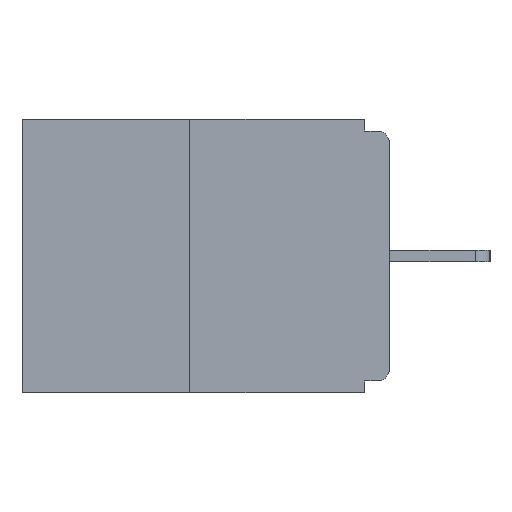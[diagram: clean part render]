
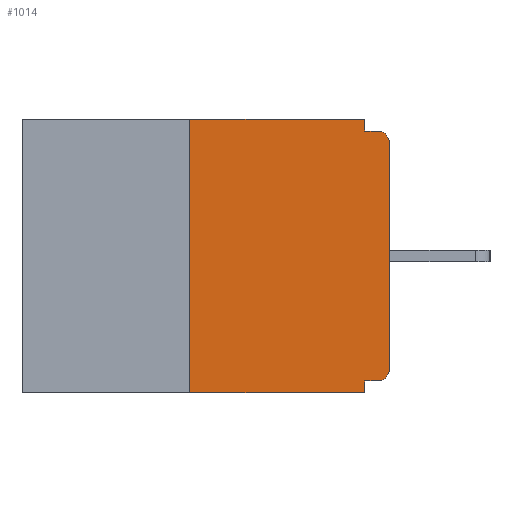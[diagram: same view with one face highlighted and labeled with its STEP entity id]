
A CAD part, left-side view. The second image highlights one B-rep face of the part: STEP entity #1014.
In plain terms, the highlighted planar face has unit normal (-1, 0, 0).
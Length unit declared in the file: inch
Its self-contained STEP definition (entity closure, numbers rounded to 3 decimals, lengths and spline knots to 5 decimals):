
#24 = AXIS2_PLACEMENT_3D ( 'NONE', #11627, #16337, #543 ) ;
#31 = PLANE ( 'NONE',  #9150 ) ;
#236 = VERTEX_POINT ( 'NONE', #1816 ) ;
#464 = DIRECTION ( 'NONE',  ( 0., 1., 0. ) ) ;
#543 = DIRECTION ( 'NONE',  ( 0., 0., -1. ) ) ;
#619 = VECTOR ( 'NONE', #464, 39.37008 ) ;
#634 = ORIENTED_EDGE ( 'NONE', *, *, #17461, .F. ) ;
#799 = VECTOR ( 'NONE', #11087, 39.37008 ) ;
#919 = CARTESIAN_POINT ( 'NONE',  ( 0., 0., -0.015 ) ) ;
#1014 = ADVANCED_FACE ( 'NONE', ( #18389 ), #31, .F. ) ;
#1371 = VERTEX_POINT ( 'NONE', #19399 ) ;
#1380 = CARTESIAN_POINT ( 'NONE',  ( 0., 0.46, -0.343 ) ) ;
#1462 = CARTESIAN_POINT ( 'NONE',  ( 0., 0.031, -0.343 ) ) ;
#1732 = VECTOR ( 'NONE', #15837, 39.37008 ) ;
#1816 = CARTESIAN_POINT ( 'NONE',  ( 0., 0.015, -0.328 ) ) ;
#1890 = DIRECTION ( 'NONE',  ( 0., 0., 1. ) ) ;
#2006 = CARTESIAN_POINT ( 'NONE',  ( 0., 0., -0.328 ) ) ;
#2594 = LINE ( 'NONE', #919, #13530 ) ;
#2870 = EDGE_CURVE ( 'NONE', #16396, #18746, #8162, .T. ) ;
#2949 = CARTESIAN_POINT ( 'NONE',  ( 0., 0.46, 0. ) ) ;
#3344 = CARTESIAN_POINT ( 'NONE',  ( 0., 0.25, -0.343 ) ) ;
#4379 = DIRECTION ( 'NONE',  ( 0., -1., 0. ) ) ;
#4965 = CARTESIAN_POINT ( 'NONE',  ( 0., 0., 0. ) ) ;
#5162 = EDGE_LOOP ( 'NONE', ( #634, #14019, #11768, #8451, #11698, #6774, #19658, #11489, #8100, #15790 ) ) ;
#5183 = CARTESIAN_POINT ( 'NONE',  ( 0., 0.031, -0.015 ) ) ;
#5186 = CIRCLE ( 'NONE', #12373, 0.015 ) ;
#6774 = ORIENTED_EDGE ( 'NONE', *, *, #8392, .T. ) ;
#6930 = DIRECTION ( 'NONE',  ( 0., 0., -1. ) ) ;
#7028 = CARTESIAN_POINT ( 'NONE',  ( 0., 0.031, 0. ) ) ;
#7117 = CARTESIAN_POINT ( 'NONE',  ( 0., 0.015, -0.015 ) ) ;
#7536 = VERTEX_POINT ( 'NONE', #10332 ) ;
#7780 = CARTESIAN_POINT ( 'NONE',  ( 0., 0.46, 0. ) ) ;
#8011 = LINE ( 'NONE', #1380, #1732 ) ;
#8100 = ORIENTED_EDGE ( 'NONE', *, *, #20112, .F. ) ;
#8162 = LINE ( 'NONE', #12700, #799 ) ;
#8213 = EDGE_CURVE ( 'NONE', #1371, #7536, #9480, .T. ) ;
#8258 = VECTOR ( 'NONE', #6930, 39.37008 ) ;
#8392 = EDGE_CURVE ( 'NONE', #236, #1371, #5186, .T. ) ;
#8451 = ORIENTED_EDGE ( 'NONE', *, *, #12208, .F. ) ;
#8612 = DIRECTION ( 'NONE',  ( 0., 0., -1. ) ) ;
#8815 = CARTESIAN_POINT ( 'NONE',  ( 0., 0.031, -0.328 ) ) ;
#9036 = DIRECTION ( 'NONE',  ( 1., 0., 0. ) ) ;
#9150 = AXIS2_PLACEMENT_3D ( 'NONE', #7780, #9036, #20032 ) ;
#9480 = LINE ( 'NONE', #4965, #18611 ) ;
#9833 = VERTEX_POINT ( 'NONE', #1462 ) ;
#10052 = DIRECTION ( 'NONE',  ( 0., -1., 0. ) ) ;
#10144 = CARTESIAN_POINT ( 'NONE',  ( 0., 0.031, 0. ) ) ;
#10171 = LINE ( 'NONE', #16431, #11483 ) ;
#10332 = CARTESIAN_POINT ( 'NONE',  ( 0., 0., -0.03 ) ) ;
#10763 = VERTEX_POINT ( 'NONE', #5183 ) ;
#10832 = EDGE_CURVE ( 'NONE', #236, #18244, #15948, .T. ) ;
#11087 = DIRECTION ( 'NONE',  ( 0., 0., 1. ) ) ;
#11332 = VERTEX_POINT ( 'NONE', #10144 ) ;
#11483 = VECTOR ( 'NONE', #8612, 39.37008 ) ;
#11489 = ORIENTED_EDGE ( 'NONE', *, *, #12169, .T. ) ;
#11627 = CARTESIAN_POINT ( 'NONE',  ( 0., 0.015, -0.03 ) ) ;
#11698 = ORIENTED_EDGE ( 'NONE', *, *, #10832, .F. ) ;
#11768 = ORIENTED_EDGE ( 'NONE', *, *, #16404, .T. ) ;
#12169 = EDGE_CURVE ( 'NONE', #7536, #13231, #17032, .T. ) ;
#12208 = EDGE_CURVE ( 'NONE', #18244, #9833, #10171, .T. ) ;
#12211 = CARTESIAN_POINT ( 'NONE',  ( 0., 0.015, -0.313 ) ) ;
#12373 = AXIS2_PLACEMENT_3D ( 'NONE', #12211, #13805, #16621 ) ;
#12562 = CARTESIAN_POINT ( 'NONE',  ( 0., 0.25, 0. ) ) ;
#12700 = CARTESIAN_POINT ( 'NONE',  ( 0., 0.25, 0. ) ) ;
#13231 = VERTEX_POINT ( 'NONE', #7117 ) ;
#13530 = VECTOR ( 'NONE', #10052, 39.37008 ) ;
#13805 = DIRECTION ( 'NONE',  ( -1., 0., 0. ) ) ;
#14019 = ORIENTED_EDGE ( 'NONE', *, *, #2870, .F. ) ;
#15790 = ORIENTED_EDGE ( 'NONE', *, *, #19254, .F. ) ;
#15837 = DIRECTION ( 'NONE',  ( 0., -1., 0. ) ) ;
#15948 = LINE ( 'NONE', #2006, #619 ) ;
#16192 = LINE ( 'NONE', #7028, #8258 ) ;
#16337 = DIRECTION ( 'NONE',  ( -1., 0., 0. ) ) ;
#16396 = VERTEX_POINT ( 'NONE', #3344 ) ;
#16404 = EDGE_CURVE ( 'NONE', #16396, #9833, #8011, .T. ) ;
#16431 = CARTESIAN_POINT ( 'NONE',  ( 0., 0.031, -0.343 ) ) ;
#16621 = DIRECTION ( 'NONE',  ( 0., 0., -1. ) ) ;
#17032 = CIRCLE ( 'NONE', #24, 0.015 ) ;
#17461 = EDGE_CURVE ( 'NONE', #18746, #11332, #18420, .T. ) ;
#17502 = VECTOR ( 'NONE', #4379, 39.37008 ) ;
#18244 = VERTEX_POINT ( 'NONE', #8815 ) ;
#18389 = FACE_OUTER_BOUND ( 'NONE', #5162, .T. ) ;
#18420 = LINE ( 'NONE', #2949, #17502 ) ;
#18611 = VECTOR ( 'NONE', #1890, 39.37008 ) ;
#18746 = VERTEX_POINT ( 'NONE', #12562 ) ;
#19254 = EDGE_CURVE ( 'NONE', #11332, #10763, #16192, .T. ) ;
#19399 = CARTESIAN_POINT ( 'NONE',  ( 0., 0., -0.313 ) ) ;
#19658 = ORIENTED_EDGE ( 'NONE', *, *, #8213, .T. ) ;
#20032 = DIRECTION ( 'NONE',  ( 0., 0., -1. ) ) ;
#20112 = EDGE_CURVE ( 'NONE', #10763, #13231, #2594, .T. ) ;
